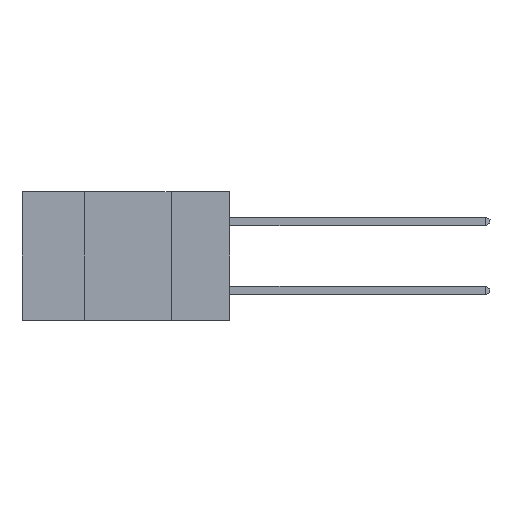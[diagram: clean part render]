
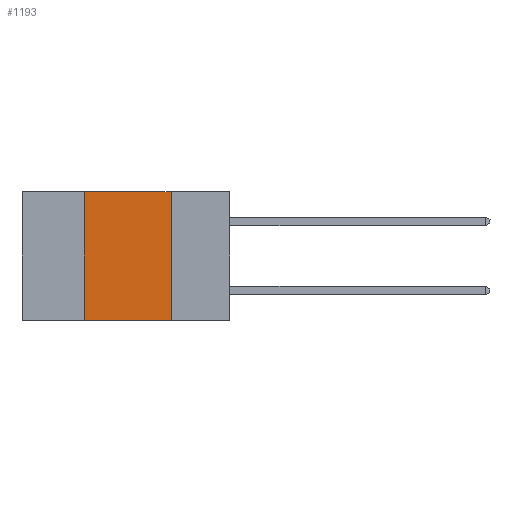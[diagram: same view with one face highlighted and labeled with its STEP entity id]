
A CAD part, left-side view. The second image highlights one B-rep face of the part: STEP entity #1193.
In plain terms, the highlighted planar face has unit normal (-1, 0, 0).
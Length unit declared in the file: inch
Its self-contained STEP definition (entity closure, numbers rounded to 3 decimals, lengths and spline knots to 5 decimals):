
#153 = PLANE ( 'NONE',  #5597 ) ;
#195 = VERTEX_POINT ( 'NONE', #9820 ) ;
#425 = ORIENTED_EDGE ( 'NONE', *, *, #4414, .T. ) ;
#587 = VECTOR ( 'NONE', #4478, 39.37008 ) ;
#862 = FACE_OUTER_BOUND ( 'NONE', #8102, .T. ) ;
#1152 = CARTESIAN_POINT ( 'NONE',  ( 0., 0.42, -0.37 ) ) ;
#1193 = ADVANCED_FACE ( 'NONE', ( #862 ), #153, .F. ) ;
#1572 = ORIENTED_EDGE ( 'NONE', *, *, #5334, .F. ) ;
#1633 = LINE ( 'NONE', #7353, #4278 ) ;
#1644 = VECTOR ( 'NONE', #9198, 39.37008 ) ;
#2522 = CARTESIAN_POINT ( 'NONE',  ( 0., 0.42, 0. ) ) ;
#2564 = CARTESIAN_POINT ( 'NONE',  ( 0., 0.6, 0. ) ) ;
#3216 = CARTESIAN_POINT ( 'NONE',  ( 0., 0.17, -0.37 ) ) ;
#4189 = DIRECTION ( 'NONE',  ( 0., 0., -1. ) ) ;
#4201 = EDGE_CURVE ( 'NONE', #195, #4533, #8561, .T. ) ;
#4278 = VECTOR ( 'NONE', #4189, 39.37008 ) ;
#4414 = EDGE_CURVE ( 'NONE', #195, #8031, #8387, .T. ) ;
#4478 = DIRECTION ( 'NONE',  ( 0., 0., 1. ) ) ;
#4533 = VERTEX_POINT ( 'NONE', #2522 ) ;
#5116 = CARTESIAN_POINT ( 'NONE',  ( 0., 0.6, -0.37 ) ) ;
#5178 = ORIENTED_EDGE ( 'NONE', *, *, #4201, .F. ) ;
#5334 = EDGE_CURVE ( 'NONE', #4533, #8884, #8200, .T. ) ;
#5597 = AXIS2_PLACEMENT_3D ( 'NONE', #2564, #9899, #6603 ) ;
#6237 = EDGE_CURVE ( 'NONE', #8884, #8031, #1633, .T. ) ;
#6481 = DIRECTION ( 'NONE',  ( 0., -1., 0. ) ) ;
#6603 = DIRECTION ( 'NONE',  ( 0., 0., -1. ) ) ;
#6998 = VECTOR ( 'NONE', #6481, 39.37008 ) ;
#7026 = CARTESIAN_POINT ( 'NONE',  ( 0., 0.17, 0. ) ) ;
#7353 = CARTESIAN_POINT ( 'NONE',  ( 0., 0.17, -0.37 ) ) ;
#8031 = VERTEX_POINT ( 'NONE', #3216 ) ;
#8102 = EDGE_LOOP ( 'NONE', ( #9429, #1572, #5178, #425 ) ) ;
#8200 = LINE ( 'NONE', #9123, #6998 ) ;
#8387 = LINE ( 'NONE', #5116, #1644 ) ;
#8561 = LINE ( 'NONE', #1152, #587 ) ;
#8884 = VERTEX_POINT ( 'NONE', #7026 ) ;
#9123 = CARTESIAN_POINT ( 'NONE',  ( 0., 0.6, 0. ) ) ;
#9198 = DIRECTION ( 'NONE',  ( 0., -1., 0. ) ) ;
#9429 = ORIENTED_EDGE ( 'NONE', *, *, #6237, .F. ) ;
#9820 = CARTESIAN_POINT ( 'NONE',  ( 0., 0.42, -0.37 ) ) ;
#9899 = DIRECTION ( 'NONE',  ( 1., 0., 0. ) ) ;
